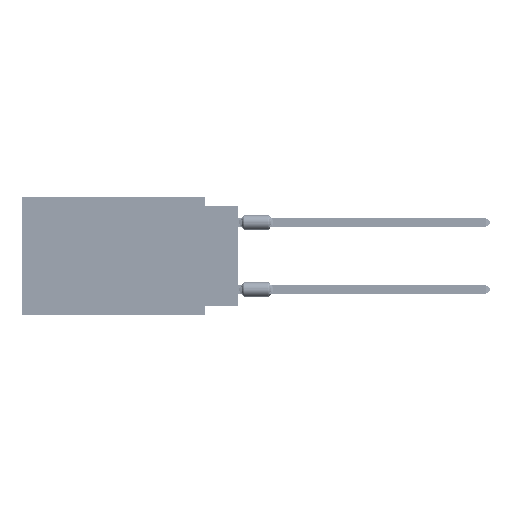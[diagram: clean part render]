
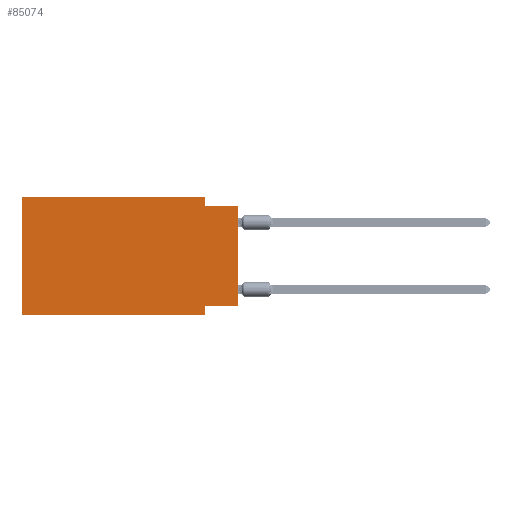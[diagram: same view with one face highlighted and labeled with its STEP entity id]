
A CAD part, left-side view. The second image highlights one B-rep face of the part: STEP entity #85074.
In plain terms, the highlighted planar face has unit normal (-1, 0, 0).
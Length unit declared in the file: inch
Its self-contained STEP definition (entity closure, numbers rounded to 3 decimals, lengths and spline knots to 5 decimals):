
#1833 = CARTESIAN_POINT ( 'NONE',  ( 0., 0., -0.025 ) ) ;
#3738 = DIRECTION ( 'NONE',  ( 1., 0., 0. ) ) ;
#4473 = EDGE_CURVE ( 'NONE', #14371, #69884, #66574, .T. ) ;
#4780 = CARTESIAN_POINT ( 'NONE',  ( 0., 0., -0.325 ) ) ;
#6366 = ORIENTED_EDGE ( 'NONE', *, *, #100416, .F. ) ;
#8280 = VERTEX_POINT ( 'NONE', #107886 ) ;
#10465 = EDGE_CURVE ( 'NONE', #14371, #8280, #41771, .T. ) ;
#14321 = DIRECTION ( 'NONE',  ( 0., -1., 0. ) ) ;
#14371 = VERTEX_POINT ( 'NONE', #69028 ) ;
#16199 = ORIENTED_EDGE ( 'NONE', *, *, #47559, .F. ) ;
#17343 = CARTESIAN_POINT ( 'NONE',  ( 0., 0., -0.325 ) ) ;
#17493 = VERTEX_POINT ( 'NONE', #63355 ) ;
#20348 = PLANE ( 'NONE',  #20776 ) ;
#20776 = AXIS2_PLACEMENT_3D ( 'NONE', #54097, #3738, #36411 ) ;
#21928 = LINE ( 'NONE', #4780, #40826 ) ;
#22400 = VECTOR ( 'NONE', #91941, 39.37008 ) ;
#22499 = LINE ( 'NONE', #56248, #97877 ) ;
#28443 = EDGE_LOOP ( 'NONE', ( #80707, #87108, #47563, #16199, #106452, #32402, #48404, #6366 ) ) ;
#31198 = DIRECTION ( 'NONE',  ( 0., 0., 1. ) ) ;
#31658 = CARTESIAN_POINT ( 'NONE',  ( 0., 0.1, 0. ) ) ;
#32402 = ORIENTED_EDGE ( 'NONE', *, *, #10465, .T. ) ;
#32412 = DIRECTION ( 'NONE',  ( 0., 0., 1. ) ) ;
#36380 = VERTEX_POINT ( 'NONE', #58325 ) ;
#36411 = DIRECTION ( 'NONE',  ( 0., 0., -1. ) ) ;
#36492 = VECTOR ( 'NONE', #92681, 39.37008 ) ;
#36959 = FACE_OUTER_BOUND ( 'NONE', #28443, .T. ) ;
#38052 = VECTOR ( 'NONE', #32412, 39.37008 ) ;
#39671 = EDGE_CURVE ( 'NONE', #99604, #36380, #48804, .T. ) ;
#40826 = VECTOR ( 'NONE', #71747, 39.37008 ) ;
#41771 = LINE ( 'NONE', #75545, #36492 ) ;
#47559 = EDGE_CURVE ( 'NONE', #69884, #99604, #81821, .T. ) ;
#47563 = ORIENTED_EDGE ( 'NONE', *, *, #39671, .F. ) ;
#48404 = ORIENTED_EDGE ( 'NONE', *, *, #103774, .F. ) ;
#48447 = VERTEX_POINT ( 'NONE', #17343 ) ;
#48804 = LINE ( 'NONE', #31658, #22400 ) ;
#49830 = VERTEX_POINT ( 'NONE', #1833 ) ;
#54097 = CARTESIAN_POINT ( 'NONE',  ( 0., 0.645, 0. ) ) ;
#56248 = CARTESIAN_POINT ( 'NONE',  ( 0., 0.1, -0.35 ) ) ;
#58325 = CARTESIAN_POINT ( 'NONE',  ( 0., 0.1, -0.025 ) ) ;
#59508 = LINE ( 'NONE', #84417, #38052 ) ;
#63355 = CARTESIAN_POINT ( 'NONE',  ( 0., 0.1, -0.325 ) ) ;
#65212 = CARTESIAN_POINT ( 'NONE',  ( 0., 0.645, 0. ) ) ;
#66574 = LINE ( 'NONE', #75986, #92436 ) ;
#69028 = CARTESIAN_POINT ( 'NONE',  ( 0., 0.645, -0.35 ) ) ;
#69884 = VERTEX_POINT ( 'NONE', #94169 ) ;
#71747 = DIRECTION ( 'NONE',  ( 0., 1., 0. ) ) ;
#75545 = CARTESIAN_POINT ( 'NONE',  ( 0., 0.645, -0.35 ) ) ;
#75986 = CARTESIAN_POINT ( 'NONE',  ( 0., 0.645, 0. ) ) ;
#77462 = EDGE_CURVE ( 'NONE', #48447, #49830, #59508, .T. ) ;
#77899 = VECTOR ( 'NONE', #81807, 39.37008 ) ;
#80707 = ORIENTED_EDGE ( 'NONE', *, *, #77462, .T. ) ;
#81807 = DIRECTION ( 'NONE',  ( 0., -1., 0. ) ) ;
#81821 = LINE ( 'NONE', #65212, #88419 ) ;
#84417 = CARTESIAN_POINT ( 'NONE',  ( 0., 0., 0. ) ) ;
#85074 = ADVANCED_FACE ( 'NONE', ( #36959 ), #20348, .F. ) ;
#87108 = ORIENTED_EDGE ( 'NONE', *, *, #100008, .F. ) ;
#88419 = VECTOR ( 'NONE', #14321, 39.37008 ) ;
#90007 = DIRECTION ( 'NONE',  ( 0., 0., -1. ) ) ;
#91941 = DIRECTION ( 'NONE',  ( 0., 0., -1. ) ) ;
#92436 = VECTOR ( 'NONE', #31198, 39.37008 ) ;
#92681 = DIRECTION ( 'NONE',  ( 0., -1., 0. ) ) ;
#94169 = CARTESIAN_POINT ( 'NONE',  ( 0., 0.645, 0. ) ) ;
#94612 = LINE ( 'NONE', #96791, #77899 ) ;
#96791 = CARTESIAN_POINT ( 'NONE',  ( 0., 0., -0.025 ) ) ;
#97877 = VECTOR ( 'NONE', #90007, 39.37008 ) ;
#99604 = VERTEX_POINT ( 'NONE', #106292 ) ;
#100008 = EDGE_CURVE ( 'NONE', #36380, #49830, #94612, .T. ) ;
#100416 = EDGE_CURVE ( 'NONE', #48447, #17493, #21928, .T. ) ;
#103774 = EDGE_CURVE ( 'NONE', #17493, #8280, #22499, .T. ) ;
#106292 = CARTESIAN_POINT ( 'NONE',  ( 0., 0.1, 0. ) ) ;
#106452 = ORIENTED_EDGE ( 'NONE', *, *, #4473, .F. ) ;
#107886 = CARTESIAN_POINT ( 'NONE',  ( 0., 0.1, -0.35 ) ) ;
